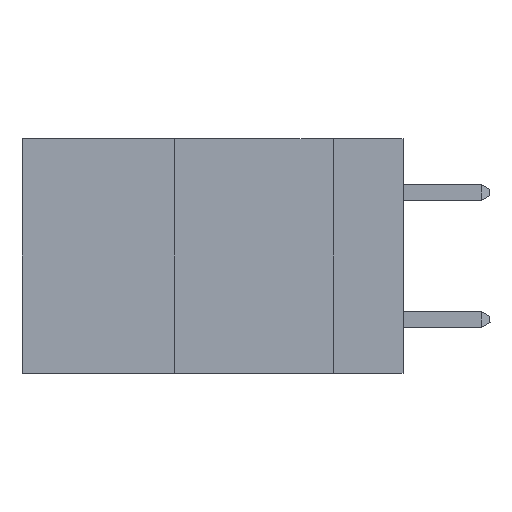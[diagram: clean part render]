
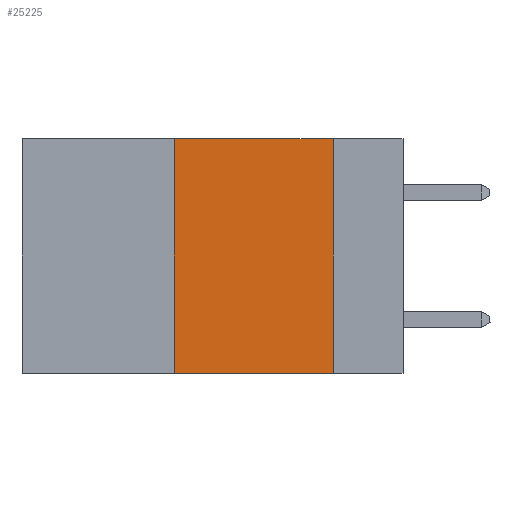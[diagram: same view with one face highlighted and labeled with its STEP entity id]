
A CAD part, left-side view. The second image highlights one B-rep face of the part: STEP entity #25225.
In plain terms, the highlighted planar face has unit normal (-1, 0, 0).
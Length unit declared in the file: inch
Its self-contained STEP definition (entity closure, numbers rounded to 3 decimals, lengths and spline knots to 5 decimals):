
#80 = EDGE_LOOP ( 'NONE', ( #8322, #16490, #17488, #24953 ) ) ;
#230 = VECTOR ( 'NONE', #12248, 39.37008 ) ;
#1301 = DIRECTION ( 'NONE',  ( 0., -1., 0. ) ) ;
#1632 = VERTEX_POINT ( 'NONE', #14013 ) ;
#1746 = DIRECTION ( 'NONE',  ( 0., -1., 0. ) ) ;
#3226 = DIRECTION ( 'NONE',  ( 0., 0., -1. ) ) ;
#3922 = VECTOR ( 'NONE', #1746, 39.37008 ) ;
#4767 = CARTESIAN_POINT ( 'NONE',  ( 0., 0.6, -0.37 ) ) ;
#5164 = VERTEX_POINT ( 'NONE', #23344 ) ;
#5931 = EDGE_CURVE ( 'NONE', #1632, #23213, #7462, .T. ) ;
#6890 = FACE_OUTER_BOUND ( 'NONE', #80, .T. ) ;
#7036 = DIRECTION ( 'NONE',  ( 0., 0., -1. ) ) ;
#7358 = CARTESIAN_POINT ( 'NONE',  ( 0., 0.6, 0. ) ) ;
#7462 = LINE ( 'NONE', #7507, #3922 ) ;
#7507 = CARTESIAN_POINT ( 'NONE',  ( 0., 0.6, 0. ) ) ;
#8322 = ORIENTED_EDGE ( 'NONE', *, *, #19666, .F. ) ;
#9098 = CARTESIAN_POINT ( 'NONE',  ( 0., 0.11, 0. ) ) ;
#10990 = CARTESIAN_POINT ( 'NONE',  ( 0., 0.11, 0. ) ) ;
#11342 = PLANE ( 'NONE',  #22391 ) ;
#12248 = DIRECTION ( 'NONE',  ( 0., 0., 1. ) ) ;
#13411 = DIRECTION ( 'NONE',  ( 1., 0., 0. ) ) ;
#14013 = CARTESIAN_POINT ( 'NONE',  ( 0., 0.36, 0. ) ) ;
#15251 = VECTOR ( 'NONE', #7036, 39.37008 ) ;
#16283 = LINE ( 'NONE', #26452, #230 ) ;
#16490 = ORIENTED_EDGE ( 'NONE', *, *, #5931, .F. ) ;
#17252 = LINE ( 'NONE', #4767, #19465 ) ;
#17488 = ORIENTED_EDGE ( 'NONE', *, *, #22930, .F. ) ;
#19465 = VECTOR ( 'NONE', #1301, 39.37008 ) ;
#19666 = EDGE_CURVE ( 'NONE', #23213, #5164, #20684, .T. ) ;
#20684 = LINE ( 'NONE', #9098, #15251 ) ;
#21236 = VERTEX_POINT ( 'NONE', #24057 ) ;
#22391 = AXIS2_PLACEMENT_3D ( 'NONE', #7358, #13411, #3226 ) ;
#22930 = EDGE_CURVE ( 'NONE', #21236, #1632, #16283, .T. ) ;
#23210 = EDGE_CURVE ( 'NONE', #21236, #5164, #17252, .T. ) ;
#23213 = VERTEX_POINT ( 'NONE', #10990 ) ;
#23344 = CARTESIAN_POINT ( 'NONE',  ( 0., 0.11, -0.37 ) ) ;
#24057 = CARTESIAN_POINT ( 'NONE',  ( 0., 0.36, -0.37 ) ) ;
#24953 = ORIENTED_EDGE ( 'NONE', *, *, #23210, .T. ) ;
#25225 = ADVANCED_FACE ( 'NONE', ( #6890 ), #11342, .F. ) ;
#26452 = CARTESIAN_POINT ( 'NONE',  ( 0., 0.36, 0. ) ) ;
